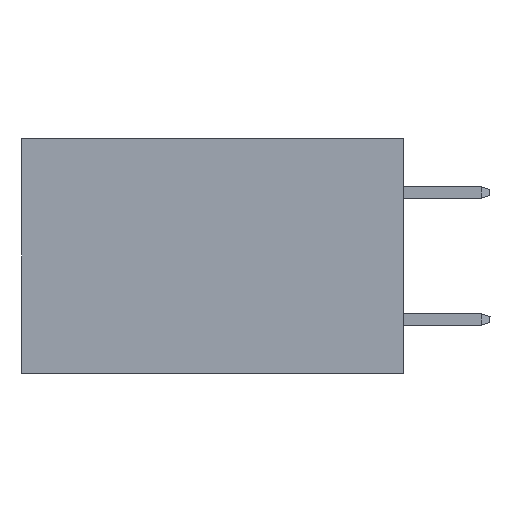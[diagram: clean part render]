
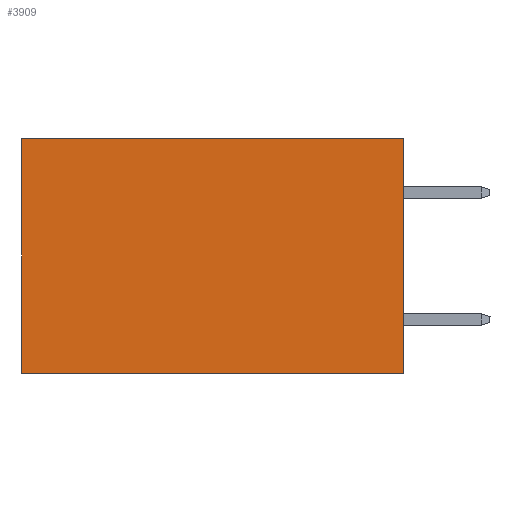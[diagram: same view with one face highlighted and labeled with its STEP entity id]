
A CAD part, left-side view. The second image highlights one B-rep face of the part: STEP entity #3909.
In plain terms, the highlighted planar face has unit normal (-1, 0, 0).
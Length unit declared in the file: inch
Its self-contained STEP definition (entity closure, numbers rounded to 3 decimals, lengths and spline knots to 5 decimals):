
#319 = VERTEX_POINT ( 'NONE', #4518 ) ;
#1145 = EDGE_CURVE ( 'NONE', #13820, #12676, #21409, .T. ) ;
#1264 = VERTEX_POINT ( 'NONE', #15659 ) ;
#3909 = ADVANCED_FACE ( 'NONE', ( #19045 ), #23869, .F. ) ;
#4518 = CARTESIAN_POINT ( 'NONE',  ( 0.2875, 0., 0. ) ) ;
#6165 = CARTESIAN_POINT ( 'NONE',  ( 0.2875, 0., 0. ) ) ;
#6507 = EDGE_LOOP ( 'NONE', ( #25675, #6924, #7529, #9816 ) ) ;
#6765 = VECTOR ( 'NONE', #28419, 39.37008 ) ;
#6924 = ORIENTED_EDGE ( 'NONE', *, *, #1145, .F. ) ;
#7529 = ORIENTED_EDGE ( 'NONE', *, *, #9054, .F. ) ;
#7807 = LINE ( 'NONE', #21108, #26363 ) ;
#9054 = EDGE_CURVE ( 'NONE', #319, #13820, #7807, .T. ) ;
#9816 = ORIENTED_EDGE ( 'NONE', *, *, #27708, .T. ) ;
#10294 = DIRECTION ( 'NONE',  ( 0., 1., 0. ) ) ;
#11079 = CARTESIAN_POINT ( 'NONE',  ( 0.2875, 0.6, 0. ) ) ;
#11276 = AXIS2_PLACEMENT_3D ( 'NONE', #6165, #23568, #28387 ) ;
#12676 = VERTEX_POINT ( 'NONE', #13606 ) ;
#12878 = VECTOR ( 'NONE', #27004, 39.37008 ) ;
#13606 = CARTESIAN_POINT ( 'NONE',  ( 0.2875, 0.6, -0.37 ) ) ;
#13663 = EDGE_CURVE ( 'NONE', #1264, #12676, #24523, .T. ) ;
#13820 = VERTEX_POINT ( 'NONE', #18510 ) ;
#13988 = VECTOR ( 'NONE', #10294, 39.37008 ) ;
#15393 = LINE ( 'NONE', #21977, #6765 ) ;
#15659 = CARTESIAN_POINT ( 'NONE',  ( 0.2875, 0.6, 0. ) ) ;
#17289 = CARTESIAN_POINT ( 'NONE',  ( 0.2875, 0., -0.37 ) ) ;
#18510 = CARTESIAN_POINT ( 'NONE',  ( 0.2875, 0., -0.37 ) ) ;
#19045 = FACE_OUTER_BOUND ( 'NONE', #6507, .T. ) ;
#21108 = CARTESIAN_POINT ( 'NONE',  ( 0.2875, 0., 0. ) ) ;
#21252 = DIRECTION ( 'NONE',  ( 0., 0., -1. ) ) ;
#21409 = LINE ( 'NONE', #17289, #13988 ) ;
#21977 = CARTESIAN_POINT ( 'NONE',  ( 0.2875, 0., 0. ) ) ;
#23568 = DIRECTION ( 'NONE',  ( 1., 0., 0. ) ) ;
#23869 = PLANE ( 'NONE',  #11276 ) ;
#24523 = LINE ( 'NONE', #11079, #12878 ) ;
#25675 = ORIENTED_EDGE ( 'NONE', *, *, #13663, .T. ) ;
#26363 = VECTOR ( 'NONE', #21252, 39.37008 ) ;
#27004 = DIRECTION ( 'NONE',  ( 0., 0., -1. ) ) ;
#27708 = EDGE_CURVE ( 'NONE', #319, #1264, #15393, .T. ) ;
#28387 = DIRECTION ( 'NONE',  ( 0., 0., -1. ) ) ;
#28419 = DIRECTION ( 'NONE',  ( 0., 1., 0. ) ) ;
